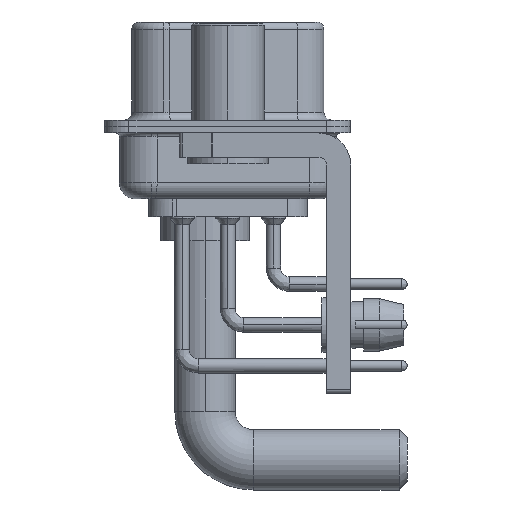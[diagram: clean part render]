
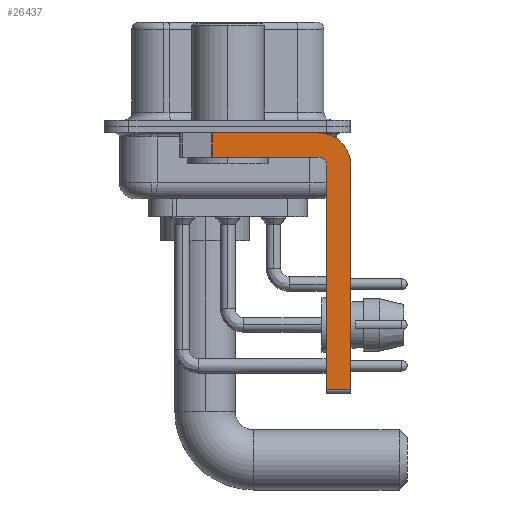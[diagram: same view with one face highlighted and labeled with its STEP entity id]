
A CAD part, left-side view. The second image highlights one B-rep face of the part: STEP entity #26437.
In plain terms, the highlighted planar face has unit normal (-1, 0, 0).
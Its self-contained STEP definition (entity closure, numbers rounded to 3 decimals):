
#636 = AXIS2_PLACEMENT_3D ( 'NONE', #12812, #6919, #35471 ) ;
#1467 = CARTESIAN_POINT ( 'NONE',  ( -2.9, 0.978, -0.4 ) ) ;
#1855 = EDGE_CURVE ( 'NONE', #16227, #16068, #7135, .T. ) ;
#2203 = VERTEX_POINT ( 'NONE', #23605 ) ;
#3304 = DIRECTION ( 'NONE',  ( -1., 0., 0. ) ) ;
#4124 = EDGE_LOOP ( 'NONE', ( #17758, #17700, #15408, #34895, #9025, #26761, #38359, #28332 ) ) ;
#4154 = LINE ( 'NONE', #26408, #36596 ) ;
#4715 = DIRECTION ( 'NONE',  ( 0., 1., 0. ) ) ;
#4752 = PLANE ( 'NONE',  #24765 ) ;
#6882 = DIRECTION ( 'NONE',  ( 0., 0., 1. ) ) ;
#6919 = DIRECTION ( 'NONE',  ( 1., 0., 0. ) ) ;
#7135 = LINE ( 'NONE', #20746, #39736 ) ;
#7640 = VERTEX_POINT ( 'NONE', #35864 ) ;
#7810 = EDGE_CURVE ( 'NONE', #2203, #29899, #34164, .T. ) ;
#8084 = CARTESIAN_POINT ( 'NONE',  ( -2.9, -5.65, -2.4 ) ) ;
#9025 = ORIENTED_EDGE ( 'NONE', *, *, #21457, .F. ) ;
#10466 = DIRECTION ( 'NONE',  ( 0., -1., 0. ) ) ;
#12734 = LINE ( 'NONE', #16089, #37283 ) ;
#12812 = CARTESIAN_POINT ( 'NONE',  ( -2.9, -5.65, -2.4 ) ) ;
#15408 = ORIENTED_EDGE ( 'NONE', *, *, #18816, .F. ) ;
#16068 = VERTEX_POINT ( 'NONE', #16610 ) ;
#16089 = CARTESIAN_POINT ( 'NONE',  ( -2.9, -7.65, -2.4 ) ) ;
#16227 = VERTEX_POINT ( 'NONE', #1467 ) ;
#16610 = CARTESIAN_POINT ( 'NONE',  ( -2.9, -5.65, -0.4 ) ) ;
#16870 = EDGE_CURVE ( 'NONE', #23845, #31052, #12734, .T. ) ;
#17700 = ORIENTED_EDGE ( 'NONE', *, *, #26769, .T. ) ;
#17758 = ORIENTED_EDGE ( 'NONE', *, *, #1855, .F. ) ;
#18733 = CIRCLE ( 'NONE', #636, 2. ) ;
#18816 = EDGE_CURVE ( 'NONE', #29899, #7640, #27790, .T. ) ;
#20746 = CARTESIAN_POINT ( 'NONE',  ( -2.9, 3., -0.4 ) ) ;
#20925 = CARTESIAN_POINT ( 'NONE',  ( -2.9, -5.65, -2.4 ) ) ;
#21367 = EDGE_CURVE ( 'NONE', #28299, #31052, #4154, .T. ) ;
#21457 = EDGE_CURVE ( 'NONE', #28299, #2203, #26000, .T. ) ;
#22150 = LINE ( 'NONE', #39166, #38177 ) ;
#22440 = CARTESIAN_POINT ( 'NONE',  ( -2.9, -7.65, -16.35 ) ) ;
#23605 = CARTESIAN_POINT ( 'NONE',  ( -2.9, -6.15, -2.4 ) ) ;
#23845 = VERTEX_POINT ( 'NONE', #38269 ) ;
#24765 = AXIS2_PLACEMENT_3D ( 'NONE', #8084, #37058, #36657 ) ;
#26000 = LINE ( 'NONE', #38374, #40647 ) ;
#26408 = CARTESIAN_POINT ( 'NONE',  ( -2.9, -5.65, -16.35 ) ) ;
#26437 = ADVANCED_FACE ( 'NONE', ( #36856 ), #4752, .F. ) ;
#26761 = ORIENTED_EDGE ( 'NONE', *, *, #21367, .T. ) ;
#26769 = EDGE_CURVE ( 'NONE', #16227, #7640, #22150, .T. ) ;
#27783 = EDGE_CURVE ( 'NONE', #16068, #23845, #18733, .T. ) ;
#27790 = LINE ( 'NONE', #30304, #33078 ) ;
#28299 = VERTEX_POINT ( 'NONE', #29333 ) ;
#28332 = ORIENTED_EDGE ( 'NONE', *, *, #27783, .F. ) ;
#29333 = CARTESIAN_POINT ( 'NONE',  ( -2.9, -6.15, -16.35 ) ) ;
#29899 = VERTEX_POINT ( 'NONE', #39607 ) ;
#30304 = CARTESIAN_POINT ( 'NONE',  ( -2.9, -5.65, -1.9 ) ) ;
#31052 = VERTEX_POINT ( 'NONE', #22440 ) ;
#32230 = DIRECTION ( 'NONE',  ( 0., 0., -1. ) ) ;
#32636 = DIRECTION ( 'NONE',  ( 0., 0., -1. ) ) ;
#33078 = VECTOR ( 'NONE', #4715, 1000. ) ;
#34164 = CIRCLE ( 'NONE', #39573, 0.5 ) ;
#34895 = ORIENTED_EDGE ( 'NONE', *, *, #7810, .F. ) ;
#35196 = DIRECTION ( 'NONE',  ( 0., 0., 1. ) ) ;
#35471 = DIRECTION ( 'NONE',  ( 0., 0., -1. ) ) ;
#35864 = CARTESIAN_POINT ( 'NONE',  ( -2.9, 0.978, -1.9 ) ) ;
#36596 = VECTOR ( 'NONE', #10466, 1000. ) ;
#36657 = DIRECTION ( 'NONE',  ( 0., 0., -1. ) ) ;
#36856 = FACE_OUTER_BOUND ( 'NONE', #4124, .T. ) ;
#37058 = DIRECTION ( 'NONE',  ( 1., 0., 0. ) ) ;
#37283 = VECTOR ( 'NONE', #32230, 1000. ) ;
#38177 = VECTOR ( 'NONE', #32636, 1000. ) ;
#38269 = CARTESIAN_POINT ( 'NONE',  ( -2.9, -7.65, -2.4 ) ) ;
#38359 = ORIENTED_EDGE ( 'NONE', *, *, #16870, .F. ) ;
#38374 = CARTESIAN_POINT ( 'NONE',  ( -2.9, -6.15, -16.6 ) ) ;
#39166 = CARTESIAN_POINT ( 'NONE',  ( -2.9, 0.978, -1.9 ) ) ;
#39573 = AXIS2_PLACEMENT_3D ( 'NONE', #20925, #3304, #35196 ) ;
#39607 = CARTESIAN_POINT ( 'NONE',  ( -2.9, -5.65, -1.9 ) ) ;
#39736 = VECTOR ( 'NONE', #39889, 1000. ) ;
#39889 = DIRECTION ( 'NONE',  ( 0., -1., 0. ) ) ;
#40647 = VECTOR ( 'NONE', #6882, 1000. ) ;
